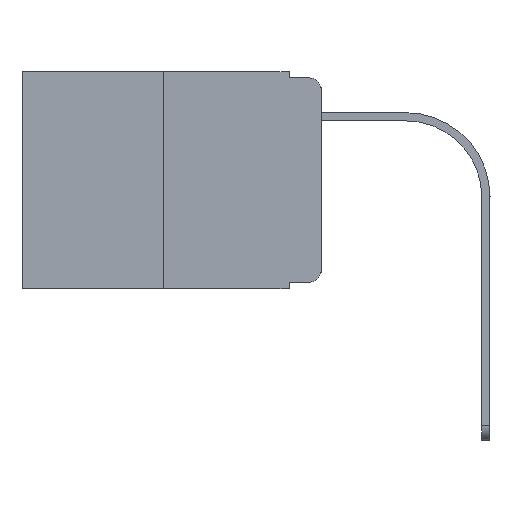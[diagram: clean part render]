
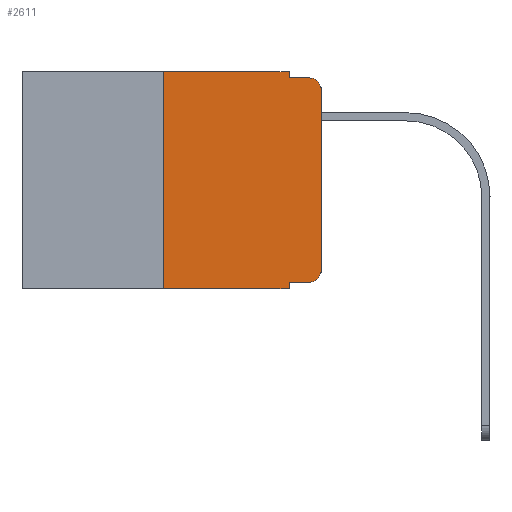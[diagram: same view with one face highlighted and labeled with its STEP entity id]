
A CAD part, left-side view. The second image highlights one B-rep face of the part: STEP entity #2611.
In plain terms, the highlighted planar face has unit normal (-1, 0, 0).
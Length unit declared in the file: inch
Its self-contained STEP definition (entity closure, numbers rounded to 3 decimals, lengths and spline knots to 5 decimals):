
#493 = CARTESIAN_POINT ( 'NONE',  ( 0., 0.02, -0.313 ) ) ;
#803 = PLANE ( 'NONE',  #14526 ) ;
#1028 = DIRECTION ( 'NONE',  ( 0., 0., -1. ) ) ;
#1067 = VECTOR ( 'NONE', #18992, 39.37008 ) ;
#2021 = ORIENTED_EDGE ( 'NONE', *, *, #19935, .F. ) ;
#2041 = EDGE_CURVE ( 'NONE', #17331, #4915, #21747, .T. ) ;
#2503 = FACE_OUTER_BOUND ( 'NONE', #20330, .T. ) ;
#2611 = ADVANCED_FACE ( 'NONE', ( #2503 ), #803, .F. ) ;
#2614 = VERTEX_POINT ( 'NONE', #19767 ) ;
#2692 = ORIENTED_EDGE ( 'NONE', *, *, #17446, .T. ) ;
#3210 = EDGE_CURVE ( 'NONE', #17331, #15510, #13625, .T. ) ;
#3673 = CIRCLE ( 'NONE', #16913, 0.02 ) ;
#3755 = CARTESIAN_POINT ( 'NONE',  ( 0., 0.051, 0. ) ) ;
#3843 = ORIENTED_EDGE ( 'NONE', *, *, #4694, .T. ) ;
#3877 = ORIENTED_EDGE ( 'NONE', *, *, #14187, .F. ) ;
#4276 = DIRECTION ( 'NONE',  ( 1., 0., 0. ) ) ;
#4694 = EDGE_CURVE ( 'NONE', #19345, #6309, #14811, .T. ) ;
#4787 = VECTOR ( 'NONE', #10046, 39.37008 ) ;
#4915 = VERTEX_POINT ( 'NONE', #6378 ) ;
#5302 = CARTESIAN_POINT ( 'NONE',  ( 0., 0., 0. ) ) ;
#5399 = CARTESIAN_POINT ( 'NONE',  ( 0., 0.473, 0. ) ) ;
#5542 = CARTESIAN_POINT ( 'NONE',  ( 0., 0.051, -0.333 ) ) ;
#5721 = CARTESIAN_POINT ( 'NONE',  ( 0., 0.02, -0.03 ) ) ;
#6126 = VERTEX_POINT ( 'NONE', #18174 ) ;
#6309 = VERTEX_POINT ( 'NONE', #18606 ) ;
#6378 = CARTESIAN_POINT ( 'NONE',  ( 0., 0.051, -0.343 ) ) ;
#7071 = VERTEX_POINT ( 'NONE', #16650 ) ;
#7141 = CARTESIAN_POINT ( 'NONE',  ( 0., 0.051, -0.01 ) ) ;
#7330 = DIRECTION ( 'NONE',  ( 0., 0., -1. ) ) ;
#7337 = VERTEX_POINT ( 'NONE', #14606 ) ;
#7603 = ORIENTED_EDGE ( 'NONE', *, *, #16767, .F. ) ;
#8639 = CARTESIAN_POINT ( 'NONE',  ( 0., 0., -0.03 ) ) ;
#8891 = ORIENTED_EDGE ( 'NONE', *, *, #13172, .T. ) ;
#9525 = VERTEX_POINT ( 'NONE', #17890 ) ;
#9792 = CARTESIAN_POINT ( 'NONE',  ( 0., 0.473, -0.343 ) ) ;
#9895 = DIRECTION ( 'NONE',  ( 0., -1., 0. ) ) ;
#10046 = DIRECTION ( 'NONE',  ( 0., -1., 0. ) ) ;
#10138 = DIRECTION ( 'NONE',  ( 0., 0., -1. ) ) ;
#10260 = LINE ( 'NONE', #7141, #11743 ) ;
#10851 = DIRECTION ( 'NONE',  ( 0., 0., -1. ) ) ;
#11198 = ORIENTED_EDGE ( 'NONE', *, *, #3210, .T. ) ;
#11607 = CARTESIAN_POINT ( 'NONE',  ( 0., 0.051, -0.333 ) ) ;
#11743 = VECTOR ( 'NONE', #13970, 39.37008 ) ;
#12482 = DIRECTION ( 'NONE',  ( -1., 0., 0. ) ) ;
#12952 = LINE ( 'NONE', #19373, #21171 ) ;
#13172 = EDGE_CURVE ( 'NONE', #15510, #9525, #3673, .T. ) ;
#13625 = LINE ( 'NONE', #11607, #4787 ) ;
#13713 = DIRECTION ( 'NONE',  ( 0., 0., -1. ) ) ;
#13970 = DIRECTION ( 'NONE',  ( 0., -1., 0. ) ) ;
#14050 = LINE ( 'NONE', #3755, #14083 ) ;
#14083 = VECTOR ( 'NONE', #13713, 39.37008 ) ;
#14187 = EDGE_CURVE ( 'NONE', #7337, #2614, #14050, .T. ) ;
#14526 = AXIS2_PLACEMENT_3D ( 'NONE', #5399, #4276, #1028 ) ;
#14584 = CARTESIAN_POINT ( 'NONE',  ( 0., 0.25, 0. ) ) ;
#14606 = CARTESIAN_POINT ( 'NONE',  ( 0., 0.051, 0. ) ) ;
#14811 = CIRCLE ( 'NONE', #18076, 0.02 ) ;
#15510 = VERTEX_POINT ( 'NONE', #18006 ) ;
#15822 = ORIENTED_EDGE ( 'NONE', *, *, #18983, .T. ) ;
#15922 = DIRECTION ( 'NONE',  ( -1., 0., 0. ) ) ;
#16642 = LINE ( 'NONE', #9792, #17151 ) ;
#16650 = CARTESIAN_POINT ( 'NONE',  ( 0., 0.25, 0. ) ) ;
#16767 = EDGE_CURVE ( 'NONE', #2614, #6309, #10260, .T. ) ;
#16913 = AXIS2_PLACEMENT_3D ( 'NONE', #493, #12482, #7330 ) ;
#17151 = VECTOR ( 'NONE', #9895, 39.37008 ) ;
#17304 = LINE ( 'NONE', #5302, #1067 ) ;
#17331 = VERTEX_POINT ( 'NONE', #5542 ) ;
#17446 = EDGE_CURVE ( 'NONE', #6126, #4915, #16642, .T. ) ;
#17890 = CARTESIAN_POINT ( 'NONE',  ( 0., 0., -0.313 ) ) ;
#18006 = CARTESIAN_POINT ( 'NONE',  ( 0., 0.02, -0.333 ) ) ;
#18060 = VECTOR ( 'NONE', #10138, 39.37008 ) ;
#18076 = AXIS2_PLACEMENT_3D ( 'NONE', #5721, #15922, #10851 ) ;
#18174 = CARTESIAN_POINT ( 'NONE',  ( 0., 0.25, -0.343 ) ) ;
#18369 = CARTESIAN_POINT ( 'NONE',  ( 0., 0.051, 0. ) ) ;
#18606 = CARTESIAN_POINT ( 'NONE',  ( 0., 0.02, -0.01 ) ) ;
#18617 = ORIENTED_EDGE ( 'NONE', *, *, #2041, .F. ) ;
#18983 = EDGE_CURVE ( 'NONE', #9525, #19345, #17304, .T. ) ;
#18992 = DIRECTION ( 'NONE',  ( 0., 0., 1. ) ) ;
#19345 = VERTEX_POINT ( 'NONE', #8639 ) ;
#19373 = CARTESIAN_POINT ( 'NONE',  ( 0., 0.473, 0. ) ) ;
#19705 = DIRECTION ( 'NONE',  ( 0., -1., 0. ) ) ;
#19767 = CARTESIAN_POINT ( 'NONE',  ( 0., 0.051, -0.01 ) ) ;
#19881 = LINE ( 'NONE', #14584, #21373 ) ;
#19935 = EDGE_CURVE ( 'NONE', #7071, #7337, #12952, .T. ) ;
#19987 = DIRECTION ( 'NONE',  ( 0., 0., 1. ) ) ;
#20330 = EDGE_LOOP ( 'NONE', ( #15822, #3843, #7603, #3877, #2021, #20748, #2692, #18617, #11198, #8891 ) ) ;
#20721 = EDGE_CURVE ( 'NONE', #6126, #7071, #19881, .T. ) ;
#20748 = ORIENTED_EDGE ( 'NONE', *, *, #20721, .F. ) ;
#21171 = VECTOR ( 'NONE', #19705, 39.37008 ) ;
#21373 = VECTOR ( 'NONE', #19987, 39.37008 ) ;
#21747 = LINE ( 'NONE', #18369, #18060 ) ;
